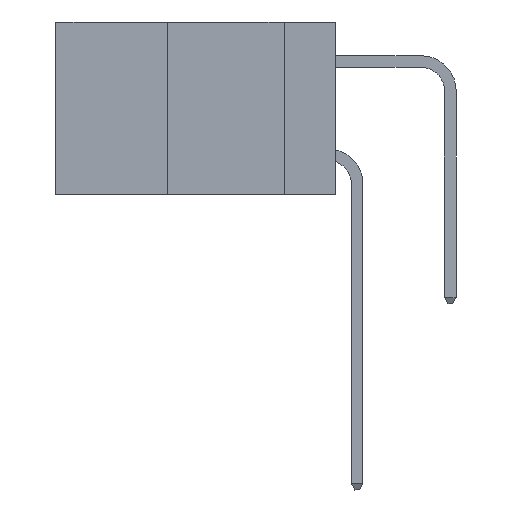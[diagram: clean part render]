
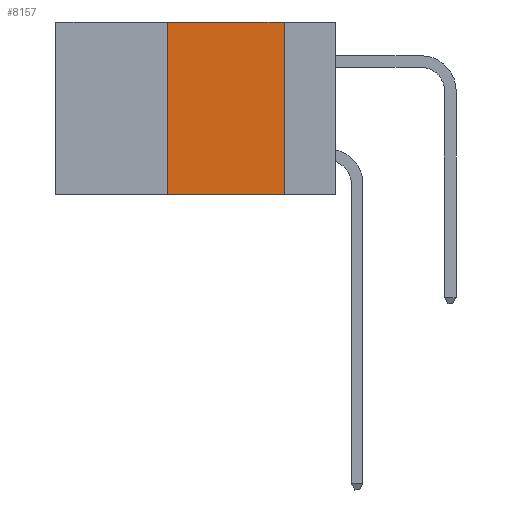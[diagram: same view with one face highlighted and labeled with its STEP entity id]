
A CAD part, left-side view. The second image highlights one B-rep face of the part: STEP entity #8157.
In plain terms, the highlighted planar face has unit normal (-1, 0, 0).
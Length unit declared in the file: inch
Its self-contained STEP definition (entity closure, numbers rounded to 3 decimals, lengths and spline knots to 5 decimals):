
#1611 = CARTESIAN_POINT ( 'NONE',  ( 0., 0.6, -0.37 ) ) ;
#2776 = DIRECTION ( 'NONE',  ( 0., 0., -1. ) ) ;
#2886 = CARTESIAN_POINT ( 'NONE',  ( 0., 0.6, 0. ) ) ;
#2946 = VECTOR ( 'NONE', #17942, 39.37008 ) ;
#4803 = EDGE_CURVE ( 'NONE', #16066, #24199, #20844, .T. ) ;
#5649 = LINE ( 'NONE', #27179, #27848 ) ;
#6158 = DIRECTION ( 'NONE',  ( 0., 0., 1. ) ) ;
#6354 = EDGE_LOOP ( 'NONE', ( #26746, #18061, #28739, #14411 ) ) ;
#8083 = VECTOR ( 'NONE', #6158, 39.37008 ) ;
#8157 = ADVANCED_FACE ( 'NONE', ( #9865 ), #16796, .F. ) ;
#9199 = LINE ( 'NONE', #29636, #2946 ) ;
#9865 = FACE_OUTER_BOUND ( 'NONE', #6354, .T. ) ;
#11362 = DIRECTION ( 'NONE',  ( 0., 0., -1. ) ) ;
#13192 = EDGE_CURVE ( 'NONE', #16066, #29886, #20435, .T. ) ;
#14411 = ORIENTED_EDGE ( 'NONE', *, *, #4803, .T. ) ;
#16066 = VERTEX_POINT ( 'NONE', #28916 ) ;
#16098 = VERTEX_POINT ( 'NONE', #26172 ) ;
#16361 = EDGE_CURVE ( 'NONE', #16098, #24199, #5649, .T. ) ;
#16796 = PLANE ( 'NONE',  #29415 ) ;
#17942 = DIRECTION ( 'NONE',  ( 0., -1., 0. ) ) ;
#18061 = ORIENTED_EDGE ( 'NONE', *, *, #28408, .F. ) ;
#20435 = LINE ( 'NONE', #22119, #8083 ) ;
#20844 = LINE ( 'NONE', #1611, #24519 ) ;
#22119 = CARTESIAN_POINT ( 'NONE',  ( 0., 0.36, 0. ) ) ;
#24199 = VERTEX_POINT ( 'NONE', #25005 ) ;
#24519 = VECTOR ( 'NONE', #25407, 39.37008 ) ;
#25005 = CARTESIAN_POINT ( 'NONE',  ( 0., 0.11, -0.37 ) ) ;
#25407 = DIRECTION ( 'NONE',  ( 0., -1., 0. ) ) ;
#25712 = CARTESIAN_POINT ( 'NONE',  ( 0., 0.36, 0. ) ) ;
#25932 = DIRECTION ( 'NONE',  ( 1., 0., 0. ) ) ;
#26172 = CARTESIAN_POINT ( 'NONE',  ( 0., 0.11, 0. ) ) ;
#26746 = ORIENTED_EDGE ( 'NONE', *, *, #16361, .F. ) ;
#27179 = CARTESIAN_POINT ( 'NONE',  ( 0., 0.11, 0. ) ) ;
#27848 = VECTOR ( 'NONE', #11362, 39.37008 ) ;
#28408 = EDGE_CURVE ( 'NONE', #29886, #16098, #9199, .T. ) ;
#28739 = ORIENTED_EDGE ( 'NONE', *, *, #13192, .F. ) ;
#28916 = CARTESIAN_POINT ( 'NONE',  ( 0., 0.36, -0.37 ) ) ;
#29415 = AXIS2_PLACEMENT_3D ( 'NONE', #2886, #25932, #2776 ) ;
#29636 = CARTESIAN_POINT ( 'NONE',  ( 0., 0.6, 0. ) ) ;
#29886 = VERTEX_POINT ( 'NONE', #25712 ) ;
